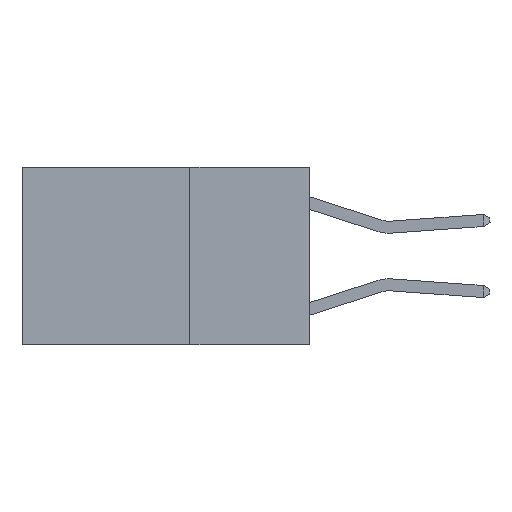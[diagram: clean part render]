
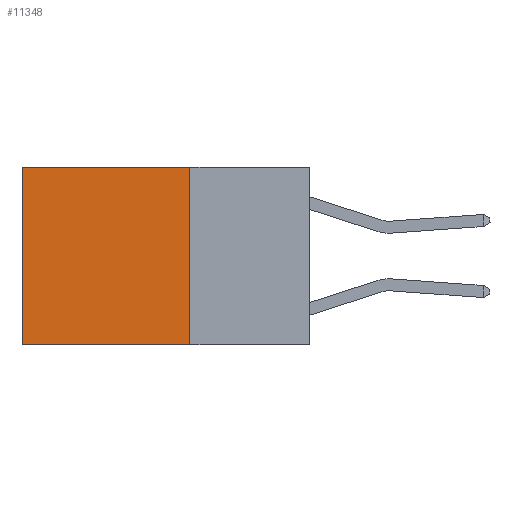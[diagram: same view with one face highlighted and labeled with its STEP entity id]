
A CAD part, left-side view. The second image highlights one B-rep face of the part: STEP entity #11348.
In plain terms, the highlighted planar face has unit normal (-1, 0, 0).
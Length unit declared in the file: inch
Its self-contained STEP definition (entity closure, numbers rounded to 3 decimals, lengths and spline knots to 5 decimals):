
#466 = VERTEX_POINT ( 'NONE', #2533 ) ;
#474 = DIRECTION ( 'NONE',  ( 1., 0., 0. ) ) ;
#1123 = CARTESIAN_POINT ( 'NONE',  ( 0.2625, 0.25, -0.37 ) ) ;
#1976 = EDGE_CURVE ( 'NONE', #3014, #4191, #4380, .T. ) ;
#1991 = EDGE_CURVE ( 'NONE', #11351, #4191, #2022, .T. ) ;
#2022 = LINE ( 'NONE', #4649, #6476 ) ;
#2533 = CARTESIAN_POINT ( 'NONE',  ( 0.2625, 0.25, 0. ) ) ;
#2693 = VECTOR ( 'NONE', #8328, 39.37008 ) ;
#2933 = DIRECTION ( 'NONE',  ( 0., 0., -1. ) ) ;
#3014 = VERTEX_POINT ( 'NONE', #5820 ) ;
#3779 = CARTESIAN_POINT ( 'NONE',  ( 0.2625, 0.25, 0. ) ) ;
#4191 = VERTEX_POINT ( 'NONE', #8542 ) ;
#4380 = LINE ( 'NONE', #1123, #9161 ) ;
#4649 = CARTESIAN_POINT ( 'NONE',  ( 0.2625, 0.6, 0. ) ) ;
#4803 = ORIENTED_EDGE ( 'NONE', *, *, #1991, .T. ) ;
#5078 = AXIS2_PLACEMENT_3D ( 'NONE', #5838, #474, #6730 ) ;
#5820 = CARTESIAN_POINT ( 'NONE',  ( 0.2625, 0.25, -0.37 ) ) ;
#5838 = CARTESIAN_POINT ( 'NONE',  ( 0.2625, 0.25, 0. ) ) ;
#6080 = ORIENTED_EDGE ( 'NONE', *, *, #9238, .F. ) ;
#6096 = ORIENTED_EDGE ( 'NONE', *, *, #1976, .F. ) ;
#6177 = LINE ( 'NONE', #3779, #6459 ) ;
#6459 = VECTOR ( 'NONE', #10049, 39.37008 ) ;
#6476 = VECTOR ( 'NONE', #2933, 39.37008 ) ;
#6730 = DIRECTION ( 'NONE',  ( 0., 0., -1. ) ) ;
#7368 = DIRECTION ( 'NONE',  ( 0., 1., 0. ) ) ;
#7904 = EDGE_LOOP ( 'NONE', ( #4803, #6096, #6080, #8029 ) ) ;
#8029 = ORIENTED_EDGE ( 'NONE', *, *, #8637, .T. ) ;
#8328 = DIRECTION ( 'NONE',  ( 0., 1., 0. ) ) ;
#8509 = PLANE ( 'NONE',  #5078 ) ;
#8542 = CARTESIAN_POINT ( 'NONE',  ( 0.2625, 0.6, -0.37 ) ) ;
#8637 = EDGE_CURVE ( 'NONE', #466, #11351, #9823, .T. ) ;
#9161 = VECTOR ( 'NONE', #7368, 39.37008 ) ;
#9206 = CARTESIAN_POINT ( 'NONE',  ( 0.2625, 0.25, 0. ) ) ;
#9238 = EDGE_CURVE ( 'NONE', #466, #3014, #6177, .T. ) ;
#9823 = LINE ( 'NONE', #9206, #2693 ) ;
#10049 = DIRECTION ( 'NONE',  ( 0., 0., -1. ) ) ;
#10493 = FACE_OUTER_BOUND ( 'NONE', #7904, .T. ) ;
#11212 = CARTESIAN_POINT ( 'NONE',  ( 0.2625, 0.6, 0. ) ) ;
#11348 = ADVANCED_FACE ( 'NONE', ( #10493 ), #8509, .F. ) ;
#11351 = VERTEX_POINT ( 'NONE', #11212 ) ;
